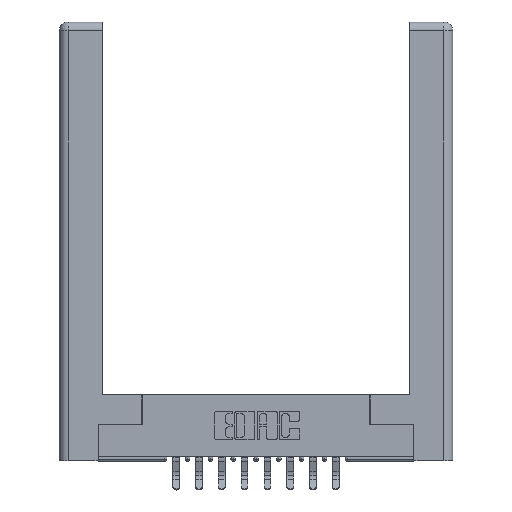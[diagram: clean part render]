
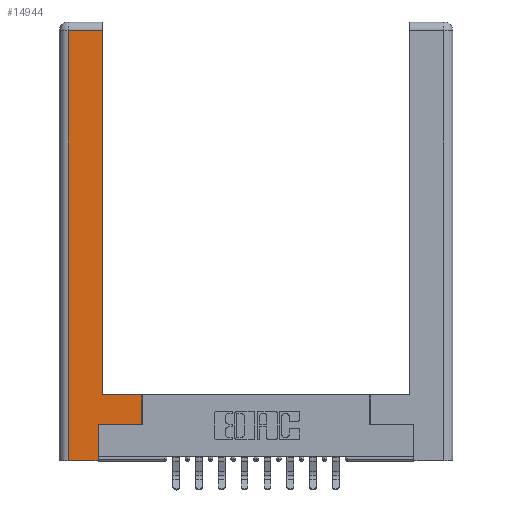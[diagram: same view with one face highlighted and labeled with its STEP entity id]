
A CAD part, top view. The second image highlights one B-rep face of the part: STEP entity #14944.
In plain terms, the highlighted planar face has unit normal (0, 0, 1).
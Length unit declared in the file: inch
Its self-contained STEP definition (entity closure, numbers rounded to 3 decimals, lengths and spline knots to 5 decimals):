
#435 = VERTEX_POINT ( 'NONE', #11724 ) ;
#620 = DIRECTION ( 'NONE',  ( 0., 1., 0. ) ) ;
#901 = VERTEX_POINT ( 'NONE', #14563 ) ;
#962 = VECTOR ( 'NONE', #5334, 39.37008 ) ;
#1217 = VECTOR ( 'NONE', #7379, 39.37008 ) ;
#1260 = CARTESIAN_POINT ( 'NONE',  ( 0.295, 3., 0. ) ) ;
#1519 = PLANE ( 'NONE',  #13563 ) ;
#1899 = VECTOR ( 'NONE', #620, 39.37008 ) ;
#2198 = VERTEX_POINT ( 'NONE', #10362 ) ;
#2449 = ORIENTED_EDGE ( 'NONE', *, *, #12548, .T. ) ;
#2561 = EDGE_CURVE ( 'NONE', #2198, #4664, #5750, .T. ) ;
#3777 = ORIENTED_EDGE ( 'NONE', *, *, #2561, .T. ) ;
#3939 = VERTEX_POINT ( 'NONE', #7889 ) ;
#4072 = ORIENTED_EDGE ( 'NONE', *, *, #5671, .T. ) ;
#4108 = DIRECTION ( 'NONE',  ( -1., 0., 0. ) ) ;
#4109 = LINE ( 'NONE', #1260, #4495 ) ;
#4263 = CARTESIAN_POINT ( 'NONE',  ( 0.265, 0., 0. ) ) ;
#4436 = ORIENTED_EDGE ( 'NONE', *, *, #14004, .T. ) ;
#4495 = VECTOR ( 'NONE', #5228, 39.37008 ) ;
#4539 = EDGE_CURVE ( 'NONE', #901, #11162, #5126, .T. ) ;
#4578 = LINE ( 'NONE', #14064, #4960 ) ;
#4664 = VERTEX_POINT ( 'NONE', #4263 ) ;
#4926 = ORIENTED_EDGE ( 'NONE', *, *, #15068, .T. ) ;
#4956 = CARTESIAN_POINT ( 'NONE',  ( 0.295, 0.45, 0. ) ) ;
#4960 = VECTOR ( 'NONE', #11549, 39.37008 ) ;
#5018 = LINE ( 'NONE', #9832, #13885 ) ;
#5126 = LINE ( 'NONE', #8940, #962 ) ;
#5167 = ORIENTED_EDGE ( 'NONE', *, *, #10996, .T. ) ;
#5228 = DIRECTION ( 'NONE',  ( 0., 1., 0. ) ) ;
#5334 = DIRECTION ( 'NONE',  ( -1., 0., 0. ) ) ;
#5390 = CARTESIAN_POINT ( 'NONE',  ( 0.265, 0.245, 0. ) ) ;
#5671 = EDGE_CURVE ( 'NONE', #10795, #435, #8536, .T. ) ;
#5750 = LINE ( 'NONE', #10864, #1217 ) ;
#6278 = CARTESIAN_POINT ( 'NONE',  ( 0.0615, 2.94, 0. ) ) ;
#7379 = DIRECTION ( 'NONE',  ( 1., 0., 0. ) ) ;
#7773 = CARTESIAN_POINT ( 'NONE',  ( 0.565, 0.245, 0. ) ) ;
#7889 = CARTESIAN_POINT ( 'NONE',  ( 0.265, 0.245, 0. ) ) ;
#8061 = EDGE_LOOP ( 'NONE', ( #5167, #8159, #2449, #3777, #4926, #11915, #4436, #4072 ) ) ;
#8159 = ORIENTED_EDGE ( 'NONE', *, *, #4539, .T. ) ;
#8536 = LINE ( 'NONE', #4956, #15478 ) ;
#8940 = CARTESIAN_POINT ( 'NONE',  ( 0.0615, 2.94, 0. ) ) ;
#9092 = CARTESIAN_POINT ( 'NONE',  ( 0.565, 0.45, 0. ) ) ;
#9832 = CARTESIAN_POINT ( 'NONE',  ( 0.0615, 0., 0. ) ) ;
#10064 = FACE_OUTER_BOUND ( 'NONE', #8061, .T. ) ;
#10362 = CARTESIAN_POINT ( 'NONE',  ( 0.0615, 0., 0. ) ) ;
#10363 = VECTOR ( 'NONE', #10950, 39.37008 ) ;
#10795 = VERTEX_POINT ( 'NONE', #9092 ) ;
#10811 = LINE ( 'NONE', #5390, #1899 ) ;
#10828 = DIRECTION ( 'NONE',  ( 0., -1., 0. ) ) ;
#10864 = CARTESIAN_POINT ( 'NONE',  ( 0.265, 0., 0. ) ) ;
#10950 = DIRECTION ( 'NONE',  ( 1., 0., 0. ) ) ;
#10996 = EDGE_CURVE ( 'NONE', #435, #901, #4109, .T. ) ;
#11147 = CARTESIAN_POINT ( 'NONE',  ( 0., 0., 0. ) ) ;
#11162 = VERTEX_POINT ( 'NONE', #6278 ) ;
#11250 = DIRECTION ( 'NONE',  ( 0., 0., -1. ) ) ;
#11549 = DIRECTION ( 'NONE',  ( 0., 1., 0. ) ) ;
#11692 = EDGE_CURVE ( 'NONE', #3939, #15608, #13173, .T. ) ;
#11724 = CARTESIAN_POINT ( 'NONE',  ( 0.295, 0.45, 0. ) ) ;
#11915 = ORIENTED_EDGE ( 'NONE', *, *, #11692, .T. ) ;
#12548 = EDGE_CURVE ( 'NONE', #11162, #2198, #5018, .T. ) ;
#13173 = LINE ( 'NONE', #13370, #10363 ) ;
#13370 = CARTESIAN_POINT ( 'NONE',  ( 0.565, 0.245, 0. ) ) ;
#13563 = AXIS2_PLACEMENT_3D ( 'NONE', #11147, #11250, #4108 ) ;
#13885 = VECTOR ( 'NONE', #10828, 39.37008 ) ;
#14004 = EDGE_CURVE ( 'NONE', #15608, #10795, #4578, .T. ) ;
#14064 = CARTESIAN_POINT ( 'NONE',  ( 0.565, 0.45, 0. ) ) ;
#14563 = CARTESIAN_POINT ( 'NONE',  ( 0.295, 2.94, 0. ) ) ;
#14595 = DIRECTION ( 'NONE',  ( -1., 0., 0. ) ) ;
#14944 = ADVANCED_FACE ( 'NONE', ( #10064 ), #1519, .F. ) ;
#15068 = EDGE_CURVE ( 'NONE', #4664, #3939, #10811, .T. ) ;
#15478 = VECTOR ( 'NONE', #14595, 39.37008 ) ;
#15608 = VERTEX_POINT ( 'NONE', #7773 ) ;
